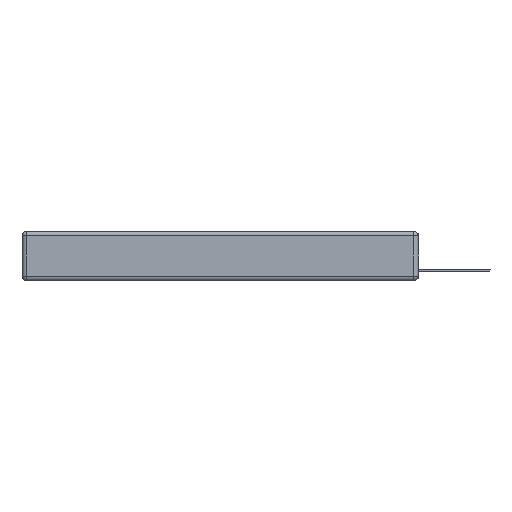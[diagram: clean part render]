
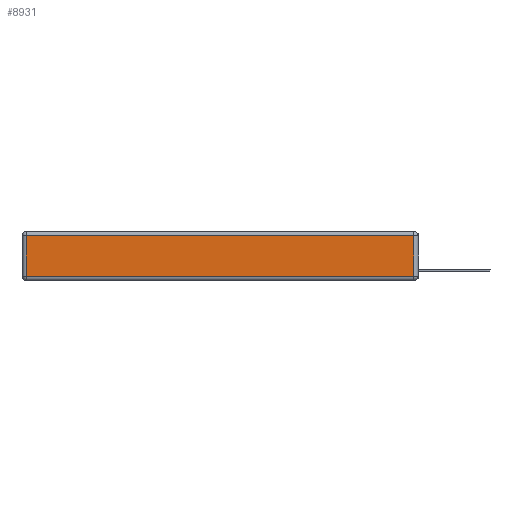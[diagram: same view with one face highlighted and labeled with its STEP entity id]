
A CAD part, left-side view. The second image highlights one B-rep face of the part: STEP entity #8931.
In plain terms, the highlighted planar face has unit normal (-1, 0, 0).
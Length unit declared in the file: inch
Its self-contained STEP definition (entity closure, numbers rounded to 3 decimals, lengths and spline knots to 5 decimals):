
#1061 = DIRECTION ( 'NONE',  ( 0., -1., 0. ) ) ;
#1245 = CARTESIAN_POINT ( 'NONE',  ( 0., 2.72, -0.343 ) ) ;
#1286 = PLANE ( 'NONE',  #15102 ) ;
#1318 = CARTESIAN_POINT ( 'NONE',  ( 0., 0.03, -0.343 ) ) ;
#1621 = CARTESIAN_POINT ( 'NONE',  ( 0., 0.03, -0.313 ) ) ;
#2601 = VECTOR ( 'NONE', #12693, 39.37008 ) ;
#4373 = DIRECTION ( 'NONE',  ( 0., 1., 0. ) ) ;
#4420 = EDGE_CURVE ( 'NONE', #15944, #24823, #8273, .T. ) ;
#4780 = ORIENTED_EDGE ( 'NONE', *, *, #4420, .T. ) ;
#5410 = EDGE_CURVE ( 'NONE', #23990, #18768, #6707, .T. ) ;
#5534 = CARTESIAN_POINT ( 'NONE',  ( 0., 2.72, -0.313 ) ) ;
#5776 = ORIENTED_EDGE ( 'NONE', *, *, #8083, .T. ) ;
#6707 = LINE ( 'NONE', #18267, #16231 ) ;
#7299 = DIRECTION ( 'NONE',  ( -1., 0., 0. ) ) ;
#7979 = EDGE_LOOP ( 'NONE', ( #15451, #24210, #4780, #5776 ) ) ;
#8083 = EDGE_CURVE ( 'NONE', #24823, #23990, #18584, .T. ) ;
#8273 = LINE ( 'NONE', #8651, #12194 ) ;
#8651 = CARTESIAN_POINT ( 'NONE',  ( 0., 2.75, -0.03 ) ) ;
#8931 = ADVANCED_FACE ( 'NONE', ( #9064 ), #1286, .T. ) ;
#9064 = FACE_OUTER_BOUND ( 'NONE', #7979, .T. ) ;
#9303 = CARTESIAN_POINT ( 'NONE',  ( 0., 0., -0.343 ) ) ;
#10014 = CARTESIAN_POINT ( 'NONE',  ( 0., 0.03, -0.03 ) ) ;
#12194 = VECTOR ( 'NONE', #4373, 39.37008 ) ;
#12693 = DIRECTION ( 'NONE',  ( 0., 0., -1. ) ) ;
#13630 = CARTESIAN_POINT ( 'NONE',  ( 0., 2.72, -0.03 ) ) ;
#14519 = LINE ( 'NONE', #1318, #23788 ) ;
#14724 = DIRECTION ( 'NONE',  ( 0., 0., 1. ) ) ;
#14754 = DIRECTION ( 'NONE',  ( 0., 0., 1. ) ) ;
#15102 = AXIS2_PLACEMENT_3D ( 'NONE', #9303, #7299, #14724 ) ;
#15451 = ORIENTED_EDGE ( 'NONE', *, *, #5410, .T. ) ;
#15944 = VERTEX_POINT ( 'NONE', #10014 ) ;
#16231 = VECTOR ( 'NONE', #1061, 39.37008 ) ;
#18267 = CARTESIAN_POINT ( 'NONE',  ( 0., 0., -0.313 ) ) ;
#18584 = LINE ( 'NONE', #1245, #2601 ) ;
#18768 = VERTEX_POINT ( 'NONE', #1621 ) ;
#23437 = EDGE_CURVE ( 'NONE', #18768, #15944, #14519, .T. ) ;
#23788 = VECTOR ( 'NONE', #14754, 39.37008 ) ;
#23990 = VERTEX_POINT ( 'NONE', #5534 ) ;
#24210 = ORIENTED_EDGE ( 'NONE', *, *, #23437, .T. ) ;
#24823 = VERTEX_POINT ( 'NONE', #13630 ) ;
